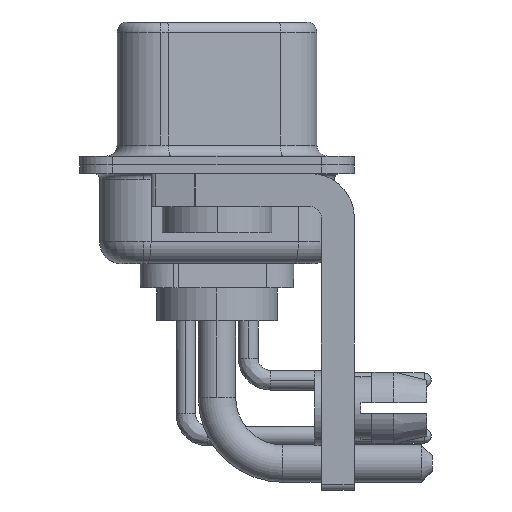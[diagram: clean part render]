
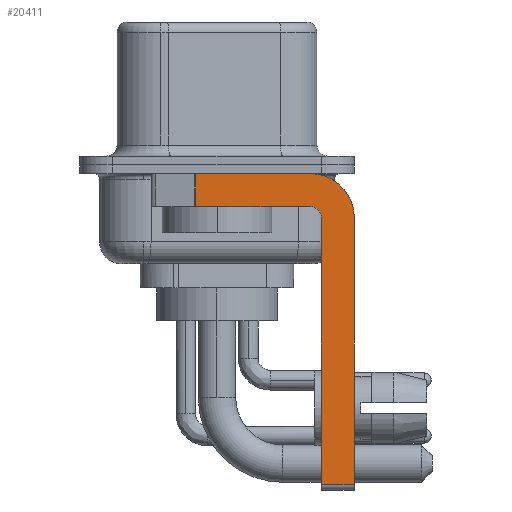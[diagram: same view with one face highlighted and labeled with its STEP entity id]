
A CAD part, left-side view. The second image highlights one B-rep face of the part: STEP entity #20411.
In plain terms, the highlighted planar face has unit normal (-1, 0, 0).
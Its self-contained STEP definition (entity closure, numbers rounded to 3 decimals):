
#65 = EDGE_CURVE ( 'NONE', #23377, #10462, #18335, .T. ) ;
#1135 = CARTESIAN_POINT ( 'NONE',  ( -2.9, -4.25, -0.4 ) ) ;
#1394 = CARTESIAN_POINT ( 'NONE',  ( -2.9, 0.978, -1.9 ) ) ;
#1800 = CARTESIAN_POINT ( 'NONE',  ( -2.9, 0.978, -0.4 ) ) ;
#2924 = DIRECTION ( 'NONE',  ( 0., 0., -1. ) ) ;
#3259 = VERTEX_POINT ( 'NONE', #14548 ) ;
#3709 = ORIENTED_EDGE ( 'NONE', *, *, #24105, .F. ) ;
#3817 = CARTESIAN_POINT ( 'NONE',  ( -2.9, -4.75, -14.8 ) ) ;
#4037 = ORIENTED_EDGE ( 'NONE', *, *, #5679, .F. ) ;
#4835 = CARTESIAN_POINT ( 'NONE',  ( -2.9, -6.25, -2.4 ) ) ;
#5075 = DIRECTION ( 'NONE',  ( 1., 0., 0. ) ) ;
#5250 = VECTOR ( 'NONE', #8616, 1000. ) ;
#5312 = VERTEX_POINT ( 'NONE', #4835 ) ;
#5410 = CIRCLE ( 'NONE', #7442, 0.5 ) ;
#5613 = LINE ( 'NONE', #13371, #13866 ) ;
#5679 = EDGE_CURVE ( 'NONE', #9411, #23240, #5410, .T. ) ;
#6786 = EDGE_CURVE ( 'NONE', #21161, #3259, #7353, .T. ) ;
#6829 = CARTESIAN_POINT ( 'NONE',  ( -2.9, -4.25, -14.55 ) ) ;
#7277 = CIRCLE ( 'NONE', #13382, 2. ) ;
#7353 = LINE ( 'NONE', #1394, #24061 ) ;
#7442 = AXIS2_PLACEMENT_3D ( 'NONE', #10408, #18108, #12813 ) ;
#8073 = DIRECTION ( 'NONE',  ( 1., 0., 0. ) ) ;
#8091 = DIRECTION ( 'NONE',  ( 0., -1., 0. ) ) ;
#8616 = DIRECTION ( 'NONE',  ( 0., -1., 0. ) ) ;
#8759 = CARTESIAN_POINT ( 'NONE',  ( -2.9, -6.25, -14.55 ) ) ;
#9411 = VERTEX_POINT ( 'NONE', #22970 ) ;
#9642 = DIRECTION ( 'NONE',  ( 0., 0., -1. ) ) ;
#10408 = CARTESIAN_POINT ( 'NONE',  ( -2.9, -4.25, -2.4 ) ) ;
#10462 = VERTEX_POINT ( 'NONE', #8759 ) ;
#10798 = CARTESIAN_POINT ( 'NONE',  ( -2.9, -4.25, -2.4 ) ) ;
#11831 = DIRECTION ( 'NONE',  ( 0., 0., 1. ) ) ;
#12581 = CARTESIAN_POINT ( 'NONE',  ( -2.9, -6.25, -2.4 ) ) ;
#12621 = EDGE_CURVE ( 'NONE', #23288, #5312, #7277, .T. ) ;
#12774 = VECTOR ( 'NONE', #2924, 1000. ) ;
#12813 = DIRECTION ( 'NONE',  ( 0., 0., 1. ) ) ;
#13025 = VECTOR ( 'NONE', #11831, 1000. ) ;
#13371 = CARTESIAN_POINT ( 'NONE',  ( -2.9, -4.25, -1.9 ) ) ;
#13382 = AXIS2_PLACEMENT_3D ( 'NONE', #21097, #8073, #23137 ) ;
#13601 = LINE ( 'NONE', #3817, #13025 ) ;
#13866 = VECTOR ( 'NONE', #23201, 1000. ) ;
#13872 = ORIENTED_EDGE ( 'NONE', *, *, #20211, .F. ) ;
#14090 = CARTESIAN_POINT ( 'NONE',  ( -2.9, -4.25, -1.9 ) ) ;
#14548 = CARTESIAN_POINT ( 'NONE',  ( -2.9, 0.978, -1.9 ) ) ;
#14725 = FACE_OUTER_BOUND ( 'NONE', #19760, .T. ) ;
#15054 = ORIENTED_EDGE ( 'NONE', *, *, #65, .T. ) ;
#15893 = AXIS2_PLACEMENT_3D ( 'NONE', #10798, #5075, #22547 ) ;
#17823 = EDGE_CURVE ( 'NONE', #23377, #9411, #13601, .T. ) ;
#17826 = LINE ( 'NONE', #21491, #19250 ) ;
#18108 = DIRECTION ( 'NONE',  ( -1., 0., 0. ) ) ;
#18335 = LINE ( 'NONE', #6829, #5250 ) ;
#18895 = ORIENTED_EDGE ( 'NONE', *, *, #17823, .F. ) ;
#19025 = ORIENTED_EDGE ( 'NONE', *, *, #24812, .F. ) ;
#19250 = VECTOR ( 'NONE', #8091, 1000. ) ;
#19760 = EDGE_LOOP ( 'NONE', ( #3709, #22335, #13872, #4037, #18895, #15054, #19025, #22035 ) ) ;
#20211 = EDGE_CURVE ( 'NONE', #23240, #3259, #5613, .T. ) ;
#20411 = ADVANCED_FACE ( 'NONE', ( #14725 ), #22419, .F. ) ;
#21097 = CARTESIAN_POINT ( 'NONE',  ( -2.9, -4.25, -2.4 ) ) ;
#21161 = VERTEX_POINT ( 'NONE', #1800 ) ;
#21491 = CARTESIAN_POINT ( 'NONE',  ( -2.9, 3., -0.4 ) ) ;
#22035 = ORIENTED_EDGE ( 'NONE', *, *, #12621, .F. ) ;
#22160 = LINE ( 'NONE', #12581, #12774 ) ;
#22265 = CARTESIAN_POINT ( 'NONE',  ( -2.9, -4.75, -14.55 ) ) ;
#22335 = ORIENTED_EDGE ( 'NONE', *, *, #6786, .T. ) ;
#22419 = PLANE ( 'NONE',  #15893 ) ;
#22547 = DIRECTION ( 'NONE',  ( 0., 0., -1. ) ) ;
#22970 = CARTESIAN_POINT ( 'NONE',  ( -2.9, -4.75, -2.4 ) ) ;
#23137 = DIRECTION ( 'NONE',  ( 0., 0., -1. ) ) ;
#23201 = DIRECTION ( 'NONE',  ( 0., 1., 0. ) ) ;
#23240 = VERTEX_POINT ( 'NONE', #14090 ) ;
#23288 = VERTEX_POINT ( 'NONE', #1135 ) ;
#23377 = VERTEX_POINT ( 'NONE', #22265 ) ;
#24061 = VECTOR ( 'NONE', #9642, 1000. ) ;
#24105 = EDGE_CURVE ( 'NONE', #21161, #23288, #17826, .T. ) ;
#24812 = EDGE_CURVE ( 'NONE', #5312, #10462, #22160, .T. ) ;
